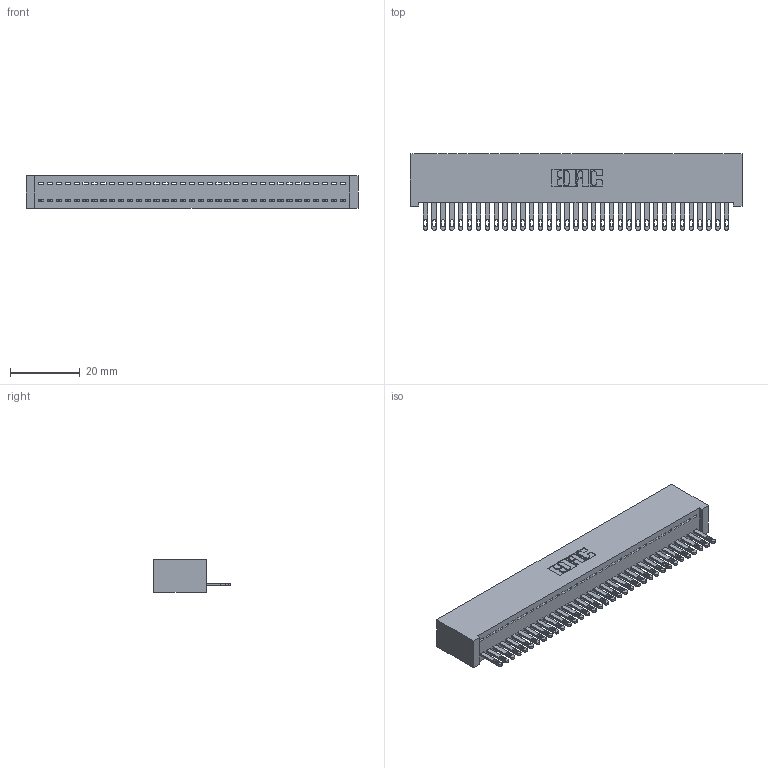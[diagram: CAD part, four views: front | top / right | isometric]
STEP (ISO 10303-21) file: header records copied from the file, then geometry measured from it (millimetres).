
FILE_DESCRIPTION (( 'STEP AP203' ), '1' );
FILE_NAME ('892-035-500-101.STEP', '2020-09-21T15:44:20', ( '' ), ( '' ), 'SwSTEP 2.0', 'SolidWorks 2020', '' );
FILE_SCHEMA (( 'CONFIG_CONTROL_DESIGN' ));
Length unit declared in the file: inch
Products named in the file (3): 345-292-001_345-293-100; 892-035-500-101; 842 Part_Lugless
Assembly tree (36 placements, depth 2):
  892-035-500-101
    842 Part_Lugless
    345-292-001_345-293-100  x35
Bounding box: 95.15 x 21.85 x 9.4 mm (x, y, z)
Volume: 8747.5 mm3; surface area: 13106.7 mm2
Topology: 36 solids, 36 shells, 1992 faces, 6155 edges, 4102 vertices
Faces by surface type: plane 1322, cylinder 670
Entity records: 21823 total; most frequent: CARTESIAN_POINT 3771, ORIENTED_EDGE 3742, DIRECTION 3189, EDGE_CURVE 1871, VECTOR 1747, LINE 1747, VERTEX_POINT 1246, AXIS2_PLACEMENT_3D 721
